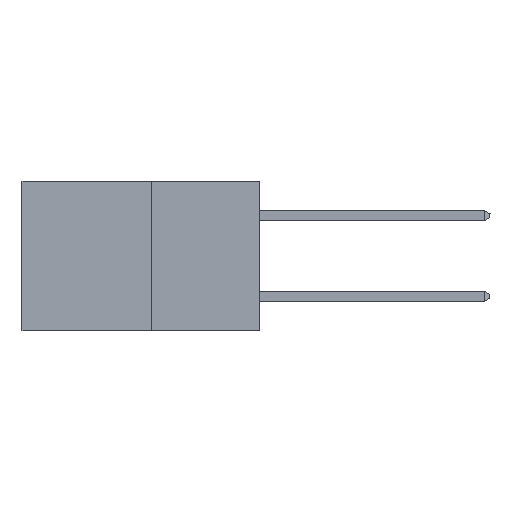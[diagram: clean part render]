
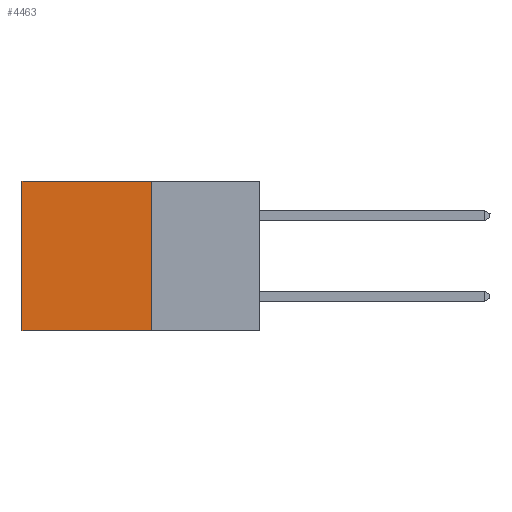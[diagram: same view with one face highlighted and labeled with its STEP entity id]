
A CAD part, left-side view. The second image highlights one B-rep face of the part: STEP entity #4463.
In plain terms, the highlighted planar face has unit normal (-1, 0, 0).
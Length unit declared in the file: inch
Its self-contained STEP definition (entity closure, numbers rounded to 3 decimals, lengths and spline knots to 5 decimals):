
#243 = CARTESIAN_POINT ( 'NONE',  ( 0.277, 0.27, -0.37 ) ) ;
#296 = VERTEX_POINT ( 'NONE', #6331 ) ;
#362 = DIRECTION ( 'NONE',  ( 0., 0., -1. ) ) ;
#1219 = CARTESIAN_POINT ( 'NONE',  ( 0.277, 0.27, 0. ) ) ;
#1696 = CARTESIAN_POINT ( 'NONE',  ( 0.277, 0.59, 0. ) ) ;
#1910 = EDGE_CURVE ( 'NONE', #3402, #7673, #2051, .T. ) ;
#2048 = EDGE_CURVE ( 'NONE', #9227, #296, #4594, .T. ) ;
#2051 = LINE ( 'NONE', #3955, #10303 ) ;
#2434 = DIRECTION ( 'NONE',  ( 0., 1., 0. ) ) ;
#2478 = DIRECTION ( 'NONE',  ( 1., 0., 0. ) ) ;
#2608 = EDGE_LOOP ( 'NONE', ( #3164, #5346, #3439, #8947 ) ) ;
#2884 = CARTESIAN_POINT ( 'NONE',  ( 0.277, 0.27, 0. ) ) ;
#2906 = FACE_OUTER_BOUND ( 'NONE', #2608, .T. ) ;
#2987 = VECTOR ( 'NONE', #2434, 39.37008 ) ;
#3098 = EDGE_CURVE ( 'NONE', #9227, #3402, #8208, .T. ) ;
#3164 = ORIENTED_EDGE ( 'NONE', *, *, #1910, .T. ) ;
#3378 = DIRECTION ( 'NONE',  ( 0., 0., -1. ) ) ;
#3402 = VERTEX_POINT ( 'NONE', #1696 ) ;
#3439 = ORIENTED_EDGE ( 'NONE', *, *, #2048, .F. ) ;
#3955 = CARTESIAN_POINT ( 'NONE',  ( 0.277, 0.59, -0.37 ) ) ;
#4228 = CARTESIAN_POINT ( 'NONE',  ( 0.277, 0.27, -0.37 ) ) ;
#4463 = ADVANCED_FACE ( 'NONE', ( #2906 ), #8530, .F. ) ;
#4594 = LINE ( 'NONE', #4228, #6755 ) ;
#5346 = ORIENTED_EDGE ( 'NONE', *, *, #8068, .F. ) ;
#6331 = CARTESIAN_POINT ( 'NONE',  ( 0.277, 0.27, -0.37 ) ) ;
#6755 = VECTOR ( 'NONE', #362, 39.37008 ) ;
#6861 = AXIS2_PLACEMENT_3D ( 'NONE', #243, #2478, #3378 ) ;
#6889 = DIRECTION ( 'NONE',  ( 0., 0., -1. ) ) ;
#7308 = CARTESIAN_POINT ( 'NONE',  ( 0.277, 0.27, -0.37 ) ) ;
#7644 = CARTESIAN_POINT ( 'NONE',  ( 0.277, 0.59, -0.37 ) ) ;
#7673 = VERTEX_POINT ( 'NONE', #7644 ) ;
#7715 = VECTOR ( 'NONE', #9151, 39.37008 ) ;
#8068 = EDGE_CURVE ( 'NONE', #296, #7673, #9592, .T. ) ;
#8208 = LINE ( 'NONE', #1219, #7715 ) ;
#8530 = PLANE ( 'NONE',  #6861 ) ;
#8947 = ORIENTED_EDGE ( 'NONE', *, *, #3098, .T. ) ;
#9151 = DIRECTION ( 'NONE',  ( 0., 1., 0. ) ) ;
#9227 = VERTEX_POINT ( 'NONE', #2884 ) ;
#9592 = LINE ( 'NONE', #7308, #2987 ) ;
#10303 = VECTOR ( 'NONE', #6889, 39.37008 ) ;
